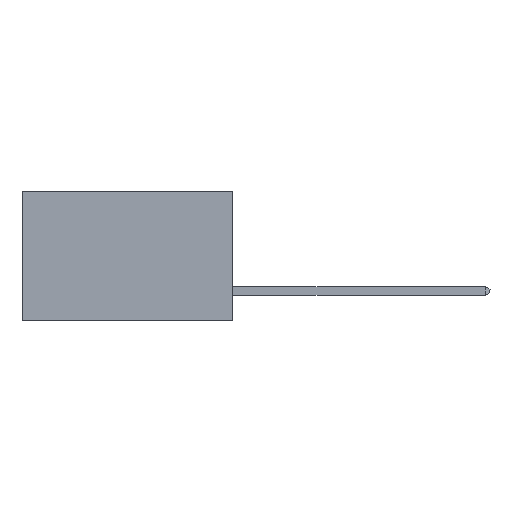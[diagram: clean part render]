
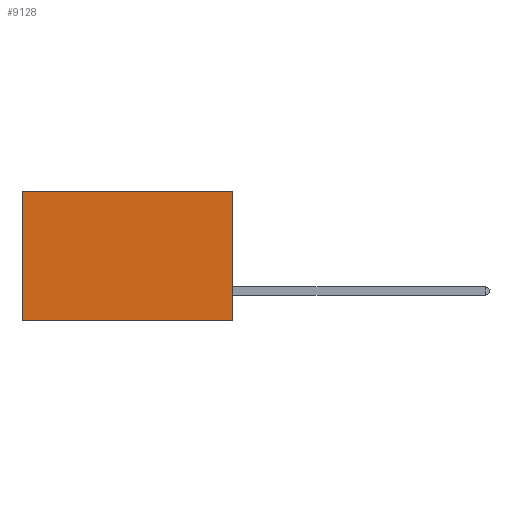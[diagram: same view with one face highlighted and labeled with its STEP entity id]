
A CAD part, left-side view. The second image highlights one B-rep face of the part: STEP entity #9128.
In plain terms, the highlighted planar face has unit normal (-1, 0, 0).
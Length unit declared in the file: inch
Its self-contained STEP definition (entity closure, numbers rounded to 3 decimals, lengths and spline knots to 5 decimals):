
#180 = EDGE_CURVE ( 'NONE', #11958, #5590, #4263, .T. ) ;
#470 = CARTESIAN_POINT ( 'NONE',  ( 0.2875, 0.6, -0.37 ) ) ;
#524 = LINE ( 'NONE', #17050, #9065 ) ;
#827 = DIRECTION ( 'NONE',  ( 1., 0., 0. ) ) ;
#1309 = VECTOR ( 'NONE', #6107, 39.37008 ) ;
#1688 = VECTOR ( 'NONE', #8096, 39.37008 ) ;
#2196 = LINE ( 'NONE', #5842, #7561 ) ;
#3175 = CARTESIAN_POINT ( 'NONE',  ( 0.2875, 0.6, 0. ) ) ;
#4263 = LINE ( 'NONE', #14946, #1688 ) ;
#4926 = LINE ( 'NONE', #3175, #1309 ) ;
#5140 = ORIENTED_EDGE ( 'NONE', *, *, #13644, .T. ) ;
#5590 = VERTEX_POINT ( 'NONE', #17749 ) ;
#5842 = CARTESIAN_POINT ( 'NONE',  ( 0.2875, 0., 0. ) ) ;
#6107 = DIRECTION ( 'NONE',  ( 0., 0., -1. ) ) ;
#6127 = FACE_OUTER_BOUND ( 'NONE', #12993, .T. ) ;
#6443 = CARTESIAN_POINT ( 'NONE',  ( 0.2875, 0., 0. ) ) ;
#6868 = VERTEX_POINT ( 'NONE', #13337 ) ;
#7561 = VECTOR ( 'NONE', #11739, 39.37008 ) ;
#7976 = AXIS2_PLACEMENT_3D ( 'NONE', #6443, #827, #8930 ) ;
#8014 = CARTESIAN_POINT ( 'NONE',  ( 0.2875, 0., 0. ) ) ;
#8096 = DIRECTION ( 'NONE',  ( 0., 0., -1. ) ) ;
#8930 = DIRECTION ( 'NONE',  ( 0., 0., -1. ) ) ;
#9065 = VECTOR ( 'NONE', #14382, 39.37008 ) ;
#9128 = ADVANCED_FACE ( 'NONE', ( #6127 ), #17220, .F. ) ;
#9586 = ORIENTED_EDGE ( 'NONE', *, *, #15569, .F. ) ;
#10644 = ORIENTED_EDGE ( 'NONE', *, *, #180, .F. ) ;
#11739 = DIRECTION ( 'NONE',  ( 0., 1., 0. ) ) ;
#11958 = VERTEX_POINT ( 'NONE', #8014 ) ;
#12715 = VERTEX_POINT ( 'NONE', #470 ) ;
#12842 = ORIENTED_EDGE ( 'NONE', *, *, #16418, .T. ) ;
#12993 = EDGE_LOOP ( 'NONE', ( #5140, #9586, #10644, #12842 ) ) ;
#13337 = CARTESIAN_POINT ( 'NONE',  ( 0.2875, 0.6, 0. ) ) ;
#13644 = EDGE_CURVE ( 'NONE', #6868, #12715, #4926, .T. ) ;
#14382 = DIRECTION ( 'NONE',  ( 0., 1., 0. ) ) ;
#14946 = CARTESIAN_POINT ( 'NONE',  ( 0.2875, 0., 0. ) ) ;
#15569 = EDGE_CURVE ( 'NONE', #5590, #12715, #524, .T. ) ;
#16418 = EDGE_CURVE ( 'NONE', #11958, #6868, #2196, .T. ) ;
#17050 = CARTESIAN_POINT ( 'NONE',  ( 0.2875, 0., -0.37 ) ) ;
#17220 = PLANE ( 'NONE',  #7976 ) ;
#17749 = CARTESIAN_POINT ( 'NONE',  ( 0.2875, 0., -0.37 ) ) ;
